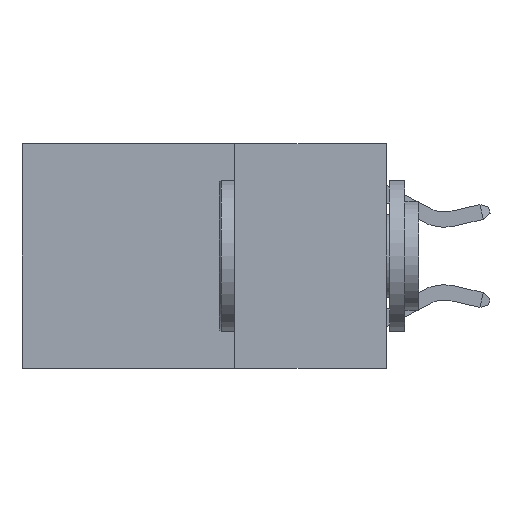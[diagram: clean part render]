
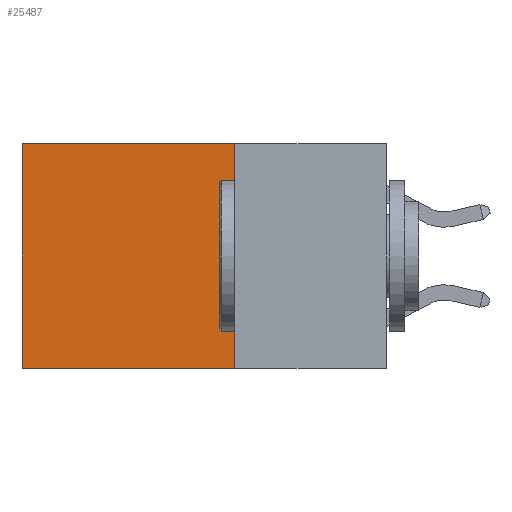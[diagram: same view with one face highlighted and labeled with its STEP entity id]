
A CAD part, left-side view. The second image highlights one B-rep face of the part: STEP entity #25487.
In plain terms, the highlighted planar face has unit normal (-1, 0, 0).
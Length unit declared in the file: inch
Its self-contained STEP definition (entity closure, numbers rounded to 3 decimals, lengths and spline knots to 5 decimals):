
#440 = CARTESIAN_POINT ( 'NONE',  ( 0.2625, 0.25, -0.37 ) ) ;
#1409 = CARTESIAN_POINT ( 'NONE',  ( 0.2625, 0.25, 0. ) ) ;
#6148 = ORIENTED_EDGE ( 'NONE', *, *, #18093, .T. ) ;
#7297 = ORIENTED_EDGE ( 'NONE', *, *, #13112, .T. ) ;
#8824 = VECTOR ( 'NONE', #21212, 39.37008 ) ;
#10541 = DIRECTION ( 'NONE',  ( 0., 0., -1. ) ) ;
#11600 = ORIENTED_EDGE ( 'NONE', *, *, #21377, .F. ) ;
#11655 = DIRECTION ( 'NONE',  ( 1., 0., 0. ) ) ;
#12226 = VECTOR ( 'NONE', #16541, 39.37008 ) ;
#12534 = LINE ( 'NONE', #1409, #18081 ) ;
#12803 = VERTEX_POINT ( 'NONE', #18897 ) ;
#13112 = EDGE_CURVE ( 'NONE', #26311, #22833, #17465, .T. ) ;
#15551 = EDGE_CURVE ( 'NONE', #24364, #22833, #27738, .T. ) ;
#16037 = FACE_OUTER_BOUND ( 'NONE', #27480, .T. ) ;
#16541 = DIRECTION ( 'NONE',  ( 0., 0., -1. ) ) ;
#16618 = CARTESIAN_POINT ( 'NONE',  ( 0.2625, 0.25, 0. ) ) ;
#16913 = PLANE ( 'NONE',  #26079 ) ;
#17465 = LINE ( 'NONE', #20659, #12226 ) ;
#17873 = LINE ( 'NONE', #16618, #8824 ) ;
#18081 = VECTOR ( 'NONE', #10541, 39.37008 ) ;
#18093 = EDGE_CURVE ( 'NONE', #12803, #26311, #17873, .T. ) ;
#18244 = CARTESIAN_POINT ( 'NONE',  ( 0.2625, 0.6, 0. ) ) ;
#18897 = CARTESIAN_POINT ( 'NONE',  ( 0.2625, 0.25, 0. ) ) ;
#18994 = DIRECTION ( 'NONE',  ( 0., 1., 0. ) ) ;
#20659 = CARTESIAN_POINT ( 'NONE',  ( 0.2625, 0.6, 0. ) ) ;
#21212 = DIRECTION ( 'NONE',  ( 0., 1., 0. ) ) ;
#21377 = EDGE_CURVE ( 'NONE', #12803, #24364, #12534, .T. ) ;
#21414 = CARTESIAN_POINT ( 'NONE',  ( 0.2625, 0.25, 0. ) ) ;
#22833 = VERTEX_POINT ( 'NONE', #27805 ) ;
#24364 = VERTEX_POINT ( 'NONE', #440 ) ;
#24851 = DIRECTION ( 'NONE',  ( 0., 0., -1. ) ) ;
#25444 = ORIENTED_EDGE ( 'NONE', *, *, #15551, .F. ) ;
#25487 = ADVANCED_FACE ( 'NONE', ( #16037 ), #16913, .F. ) ;
#26079 = AXIS2_PLACEMENT_3D ( 'NONE', #21414, #11655, #24851 ) ;
#26311 = VERTEX_POINT ( 'NONE', #18244 ) ;
#27039 = VECTOR ( 'NONE', #18994, 39.37008 ) ;
#27480 = EDGE_LOOP ( 'NONE', ( #7297, #25444, #11600, #6148 ) ) ;
#27738 = LINE ( 'NONE', #27957, #27039 ) ;
#27805 = CARTESIAN_POINT ( 'NONE',  ( 0.2625, 0.6, -0.37 ) ) ;
#27957 = CARTESIAN_POINT ( 'NONE',  ( 0.2625, 0.25, -0.37 ) ) ;
